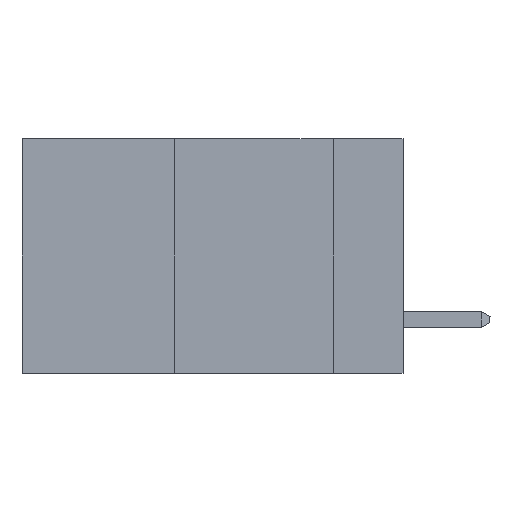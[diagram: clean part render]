
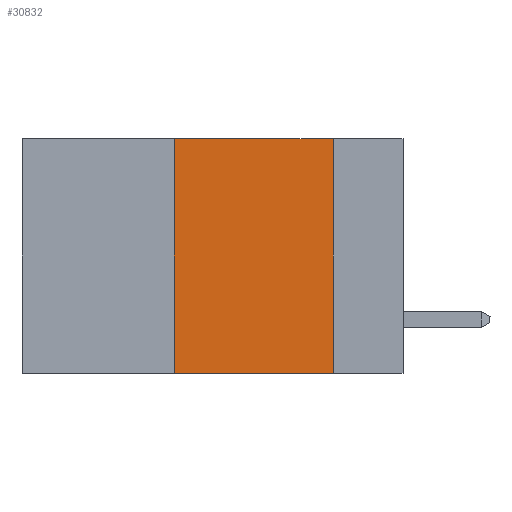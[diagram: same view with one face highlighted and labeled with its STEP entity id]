
A CAD part, left-side view. The second image highlights one B-rep face of the part: STEP entity #30832.
In plain terms, the highlighted planar face has unit normal (-1, 0, 0).
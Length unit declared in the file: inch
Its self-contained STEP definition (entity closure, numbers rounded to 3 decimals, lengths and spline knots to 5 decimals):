
#319 = DIRECTION ( 'NONE',  ( 0., 0., 1. ) ) ;
#1807 = AXIS2_PLACEMENT_3D ( 'NONE', #3343, #13351, #15656 ) ;
#2472 = VECTOR ( 'NONE', #24966, 39.37008 ) ;
#2782 = VECTOR ( 'NONE', #16026, 39.37008 ) ;
#3164 = LINE ( 'NONE', #20819, #17243 ) ;
#3343 = CARTESIAN_POINT ( 'NONE',  ( 0., 0.6, 0. ) ) ;
#5612 = CARTESIAN_POINT ( 'NONE',  ( 0., 0.36, 0. ) ) ;
#6482 = VERTEX_POINT ( 'NONE', #7530 ) ;
#7387 = VERTEX_POINT ( 'NONE', #15073 ) ;
#7530 = CARTESIAN_POINT ( 'NONE',  ( 0., 0.36, -0.37 ) ) ;
#8172 = PLANE ( 'NONE',  #1807 ) ;
#13351 = DIRECTION ( 'NONE',  ( 1., 0., 0. ) ) ;
#13363 = DIRECTION ( 'NONE',  ( 0., -1., 0. ) ) ;
#13501 = CARTESIAN_POINT ( 'NONE',  ( 0., 0.6, 0. ) ) ;
#14691 = ORIENTED_EDGE ( 'NONE', *, *, #19054, .T. ) ;
#15073 = CARTESIAN_POINT ( 'NONE',  ( 0., 0.11, 0. ) ) ;
#15156 = EDGE_CURVE ( 'NONE', #6482, #28318, #28870, .T. ) ;
#15588 = ORIENTED_EDGE ( 'NONE', *, *, #25573, .F. ) ;
#15656 = DIRECTION ( 'NONE',  ( 0., 0., -1. ) ) ;
#16026 = DIRECTION ( 'NONE',  ( 0., -1., 0. ) ) ;
#16091 = ORIENTED_EDGE ( 'NONE', *, *, #15156, .F. ) ;
#17243 = VECTOR ( 'NONE', #13363, 39.37008 ) ;
#17789 = CARTESIAN_POINT ( 'NONE',  ( 0., 0.36, 0. ) ) ;
#18959 = VERTEX_POINT ( 'NONE', #20392 ) ;
#19054 = EDGE_CURVE ( 'NONE', #6482, #18959, #3164, .T. ) ;
#19822 = ORIENTED_EDGE ( 'NONE', *, *, #26000, .F. ) ;
#20356 = EDGE_LOOP ( 'NONE', ( #15588, #19822, #16091, #14691 ) ) ;
#20392 = CARTESIAN_POINT ( 'NONE',  ( 0., 0.11, -0.37 ) ) ;
#20819 = CARTESIAN_POINT ( 'NONE',  ( 0., 0.6, -0.37 ) ) ;
#22729 = LINE ( 'NONE', #13501, #2782 ) ;
#23586 = LINE ( 'NONE', #25064, #2472 ) ;
#24966 = DIRECTION ( 'NONE',  ( 0., 0., -1. ) ) ;
#25064 = CARTESIAN_POINT ( 'NONE',  ( 0., 0.11, 0. ) ) ;
#25573 = EDGE_CURVE ( 'NONE', #7387, #18959, #23586, .T. ) ;
#26000 = EDGE_CURVE ( 'NONE', #28318, #7387, #22729, .T. ) ;
#26824 = FACE_OUTER_BOUND ( 'NONE', #20356, .T. ) ;
#26921 = VECTOR ( 'NONE', #319, 39.37008 ) ;
#28318 = VERTEX_POINT ( 'NONE', #5612 ) ;
#28870 = LINE ( 'NONE', #17789, #26921 ) ;
#30832 = ADVANCED_FACE ( 'NONE', ( #26824 ), #8172, .F. ) ;
